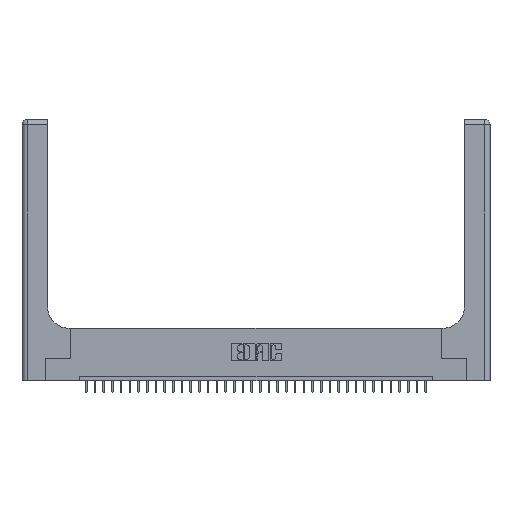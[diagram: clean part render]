
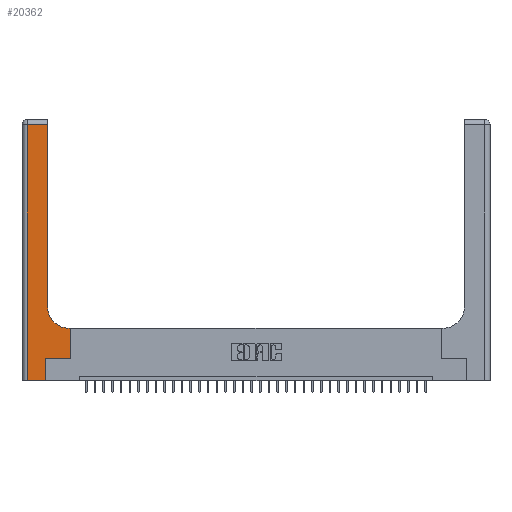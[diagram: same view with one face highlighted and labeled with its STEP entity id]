
A CAD part, top view. The second image highlights one B-rep face of the part: STEP entity #20362.
In plain terms, the highlighted planar face has unit normal (0, 0, 1).
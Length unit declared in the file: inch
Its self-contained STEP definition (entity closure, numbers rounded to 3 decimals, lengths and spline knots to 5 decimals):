
#106 = VECTOR ( 'NONE', #32346, 39.37008 ) ;
#299 = CARTESIAN_POINT ( 'NONE',  ( 0.269, 0.25, 0.37 ) ) ;
#1161 = ORIENTED_EDGE ( 'NONE', *, *, #5553, .T. ) ;
#1273 = VECTOR ( 'NONE', #21603, 39.37008 ) ;
#2208 = EDGE_LOOP ( 'NONE', ( #27302, #1161, #13367, #11765, #10141, #25100, #23145, #23511, #14310 ) ) ;
#2547 = DIRECTION ( 'NONE',  ( 0., 0., -1. ) ) ;
#2866 = DIRECTION ( 'NONE',  ( 1., 0., 0. ) ) ;
#2932 = EDGE_CURVE ( 'NONE', #31630, #31443, #18338, .T. ) ;
#3224 = CARTESIAN_POINT ( 'NONE',  ( 0.06, 3., 0.37 ) ) ;
#5056 = EDGE_CURVE ( 'NONE', #35520, #14528, #9162, .T. ) ;
#5419 = CARTESIAN_POINT ( 'NONE',  ( 0., 3., 0.37 ) ) ;
#5553 = EDGE_CURVE ( 'NONE', #15408, #35520, #10738, .T. ) ;
#6954 = EDGE_CURVE ( 'NONE', #17439, #15408, #26420, .T. ) ;
#7729 = VECTOR ( 'NONE', #25428, 39.37008 ) ;
#8214 = DIRECTION ( 'NONE',  ( -1., 0., 0. ) ) ;
#8281 = CARTESIAN_POINT ( 'NONE',  ( 0.5415, 0.85, 0.37 ) ) ;
#9162 = LINE ( 'NONE', #3224, #7729 ) ;
#9171 = DIRECTION ( 'NONE',  ( -1., 0., 0. ) ) ;
#9365 = CARTESIAN_POINT ( 'NONE',  ( 0.2915, 0.85, 0.37 ) ) ;
#10141 = ORIENTED_EDGE ( 'NONE', *, *, #29130, .T. ) ;
#10710 = VERTEX_POINT ( 'NONE', #31464 ) ;
#10738 = LINE ( 'NONE', #16167, #28551 ) ;
#11079 = LINE ( 'NONE', #13978, #19401 ) ;
#11765 = ORIENTED_EDGE ( 'NONE', *, *, #32682, .T. ) ;
#13031 = CARTESIAN_POINT ( 'NONE',  ( 0.06, 0., 0.37 ) ) ;
#13075 = CARTESIAN_POINT ( 'NONE',  ( 0.5585, 0.6, 0.37 ) ) ;
#13367 = ORIENTED_EDGE ( 'NONE', *, *, #5056, .T. ) ;
#13791 = DIRECTION ( 'NONE',  ( 1., 0., 0. ) ) ;
#13978 = CARTESIAN_POINT ( 'NONE',  ( 0., 0., 0.37 ) ) ;
#14310 = ORIENTED_EDGE ( 'NONE', *, *, #26176, .T. ) ;
#14493 = EDGE_CURVE ( 'NONE', #15693, #16353, #31818, .T. ) ;
#14528 = VERTEX_POINT ( 'NONE', #13031 ) ;
#15408 = VERTEX_POINT ( 'NONE', #26311 ) ;
#15465 = EDGE_CURVE ( 'NONE', #16353, #31630, #21778, .T. ) ;
#15693 = VERTEX_POINT ( 'NONE', #299 ) ;
#16167 = CARTESIAN_POINT ( 'NONE',  ( 0., 2.94, 0.37 ) ) ;
#16353 = VERTEX_POINT ( 'NONE', #32834 ) ;
#16444 = DIRECTION ( 'NONE',  ( -1., 0., 0. ) ) ;
#17439 = VERTEX_POINT ( 'NONE', #9365 ) ;
#18277 = CARTESIAN_POINT ( 'NONE',  ( 0.269, 0.25, 0.37 ) ) ;
#18338 = LINE ( 'NONE', #33715, #20976 ) ;
#18342 = CARTESIAN_POINT ( 'NONE',  ( 0.06, 2.94, 0.37 ) ) ;
#18388 = AXIS2_PLACEMENT_3D ( 'NONE', #8281, #19295, #2866 ) ;
#19295 = DIRECTION ( 'NONE',  ( 0., 0., -1. ) ) ;
#19401 = VECTOR ( 'NONE', #13791, 39.37008 ) ;
#19979 = VECTOR ( 'NONE', #28602, 39.37008 ) ;
#20121 = CARTESIAN_POINT ( 'NONE',  ( 0.5415, 0.6, 0.37 ) ) ;
#20362 = ADVANCED_FACE ( 'NONE', ( #29994 ), #27814, .F. ) ;
#20976 = VECTOR ( 'NONE', #9171, 39.37008 ) ;
#21603 = DIRECTION ( 'NONE',  ( 0., 1., 0. ) ) ;
#21677 = LINE ( 'NONE', #33207, #28261 ) ;
#21778 = LINE ( 'NONE', #32598, #1273 ) ;
#23145 = ORIENTED_EDGE ( 'NONE', *, *, #15465, .T. ) ;
#23511 = ORIENTED_EDGE ( 'NONE', *, *, #2932, .T. ) ;
#24537 = AXIS2_PLACEMENT_3D ( 'NONE', #5419, #2547, #16444 ) ;
#25100 = ORIENTED_EDGE ( 'NONE', *, *, #14493, .T. ) ;
#25428 = DIRECTION ( 'NONE',  ( 0., -1., 0. ) ) ;
#26176 = EDGE_CURVE ( 'NONE', #31443, #17439, #34509, .T. ) ;
#26311 = CARTESIAN_POINT ( 'NONE',  ( 0.2915, 2.94, 0.37 ) ) ;
#26420 = LINE ( 'NONE', #31838, #19979 ) ;
#27302 = ORIENTED_EDGE ( 'NONE', *, *, #6954, .T. ) ;
#27814 = PLANE ( 'NONE',  #24537 ) ;
#27815 = DIRECTION ( 'NONE',  ( 0., 1., 0. ) ) ;
#28261 = VECTOR ( 'NONE', #27815, 39.37008 ) ;
#28551 = VECTOR ( 'NONE', #8214, 39.37008 ) ;
#28602 = DIRECTION ( 'NONE',  ( 0., 1., 0. ) ) ;
#29130 = EDGE_CURVE ( 'NONE', #10710, #15693, #21677, .T. ) ;
#29994 = FACE_OUTER_BOUND ( 'NONE', #2208, .T. ) ;
#31443 = VERTEX_POINT ( 'NONE', #20121 ) ;
#31464 = CARTESIAN_POINT ( 'NONE',  ( 0.269, 0., 0.37 ) ) ;
#31630 = VERTEX_POINT ( 'NONE', #13075 ) ;
#31818 = LINE ( 'NONE', #18277, #106 ) ;
#31838 = CARTESIAN_POINT ( 'NONE',  ( 0.2915, 3., 0.37 ) ) ;
#32346 = DIRECTION ( 'NONE',  ( 1., 0., 0. ) ) ;
#32598 = CARTESIAN_POINT ( 'NONE',  ( 0.5585, 0.25, 0.37 ) ) ;
#32682 = EDGE_CURVE ( 'NONE', #14528, #10710, #11079, .T. ) ;
#32834 = CARTESIAN_POINT ( 'NONE',  ( 0.5585, 0.25, 0.37 ) ) ;
#33207 = CARTESIAN_POINT ( 'NONE',  ( 0.269, 0., 0.37 ) ) ;
#33715 = CARTESIAN_POINT ( 'NONE',  ( 0.2915, 0.6, 0.37 ) ) ;
#34509 = CIRCLE ( 'NONE', #18388, 0.25 ) ;
#35520 = VERTEX_POINT ( 'NONE', #18342 ) ;
